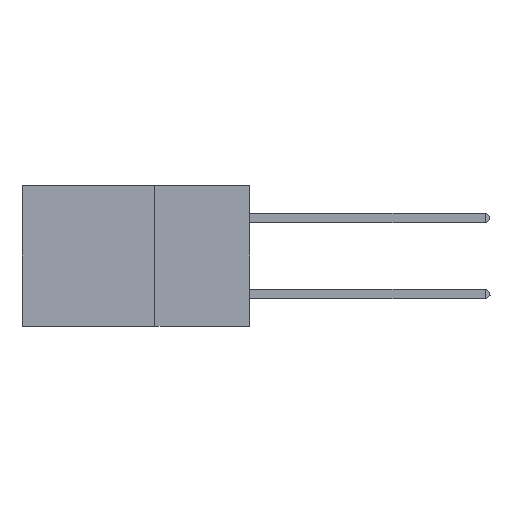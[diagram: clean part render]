
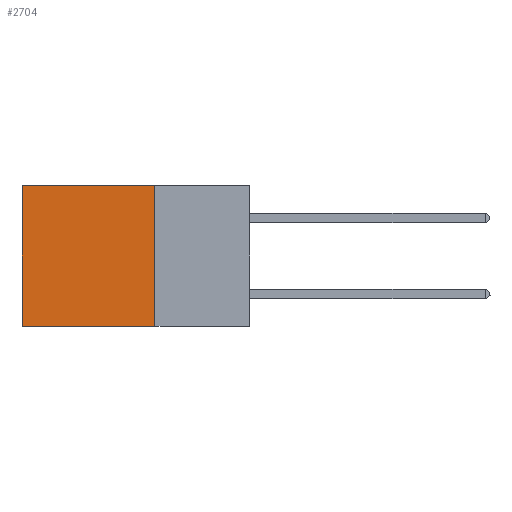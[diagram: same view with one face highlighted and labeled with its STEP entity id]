
A CAD part, left-side view. The second image highlights one B-rep face of the part: STEP entity #2704.
In plain terms, the highlighted planar face has unit normal (-1, 0, 0).
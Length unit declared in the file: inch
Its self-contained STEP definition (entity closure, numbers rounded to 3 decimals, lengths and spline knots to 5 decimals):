
#434 = CARTESIAN_POINT ( 'NONE',  ( 0.2875, 0.6, 0. ) ) ;
#1211 = EDGE_CURVE ( 'NONE', #20388, #5882, #27237, .T. ) ;
#1251 = VECTOR ( 'NONE', #1819, 39.37008 ) ;
#1439 = CARTESIAN_POINT ( 'NONE',  ( 0.2875, 0.25, 0. ) ) ;
#1819 = DIRECTION ( 'NONE',  ( 0., 1., 0. ) ) ;
#2704 = ADVANCED_FACE ( 'NONE', ( #5356 ), #8765, .F. ) ;
#5356 = FACE_OUTER_BOUND ( 'NONE', #32972, .T. ) ;
#5433 = ORIENTED_EDGE ( 'NONE', *, *, #1211, .F. ) ;
#5531 = VECTOR ( 'NONE', #13699, 39.37008 ) ;
#5635 = DIRECTION ( 'NONE',  ( 0., 0., -1. ) ) ;
#5882 = VERTEX_POINT ( 'NONE', #13797 ) ;
#8765 = PLANE ( 'NONE',  #11780 ) ;
#9101 = EDGE_CURVE ( 'NONE', #16136, #20388, #14178, .T. ) ;
#9284 = CARTESIAN_POINT ( 'NONE',  ( 0.2875, 0.25, -0.37 ) ) ;
#10305 = VERTEX_POINT ( 'NONE', #434 ) ;
#11780 = AXIS2_PLACEMENT_3D ( 'NONE', #15323, #25080, #5635 ) ;
#12382 = ORIENTED_EDGE ( 'NONE', *, *, #9101, .F. ) ;
#13699 = DIRECTION ( 'NONE',  ( 0., 0., -1. ) ) ;
#13797 = CARTESIAN_POINT ( 'NONE',  ( 0.2875, 0.6, -0.37 ) ) ;
#13920 = CARTESIAN_POINT ( 'NONE',  ( 0.2875, 0.25, 0. ) ) ;
#14178 = LINE ( 'NONE', #33047, #5531 ) ;
#14862 = LINE ( 'NONE', #38583, #38595 ) ;
#14959 = ORIENTED_EDGE ( 'NONE', *, *, #27410, .T. ) ;
#15323 = CARTESIAN_POINT ( 'NONE',  ( 0.2875, 0.25, 0. ) ) ;
#16018 = DIRECTION ( 'NONE',  ( 0., 0., -1. ) ) ;
#16136 = VERTEX_POINT ( 'NONE', #13920 ) ;
#20388 = VERTEX_POINT ( 'NONE', #9284 ) ;
#25080 = DIRECTION ( 'NONE',  ( 1., 0., 0. ) ) ;
#27237 = LINE ( 'NONE', #40656, #1251 ) ;
#27410 = EDGE_CURVE ( 'NONE', #10305, #5882, #14862, .T. ) ;
#27496 = DIRECTION ( 'NONE',  ( 0., 1., 0. ) ) ;
#32972 = EDGE_LOOP ( 'NONE', ( #14959, #5433, #12382, #34950 ) ) ;
#33047 = CARTESIAN_POINT ( 'NONE',  ( 0.2875, 0.25, 0. ) ) ;
#34950 = ORIENTED_EDGE ( 'NONE', *, *, #36043, .T. ) ;
#36043 = EDGE_CURVE ( 'NONE', #16136, #10305, #39331, .T. ) ;
#38345 = VECTOR ( 'NONE', #27496, 39.37008 ) ;
#38583 = CARTESIAN_POINT ( 'NONE',  ( 0.2875, 0.6, 0. ) ) ;
#38595 = VECTOR ( 'NONE', #16018, 39.37008 ) ;
#39331 = LINE ( 'NONE', #1439, #38345 ) ;
#40656 = CARTESIAN_POINT ( 'NONE',  ( 0.2875, 0.25, -0.37 ) ) ;
